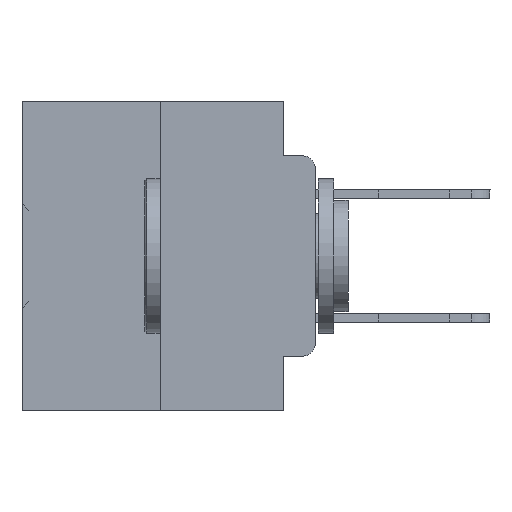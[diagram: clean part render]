
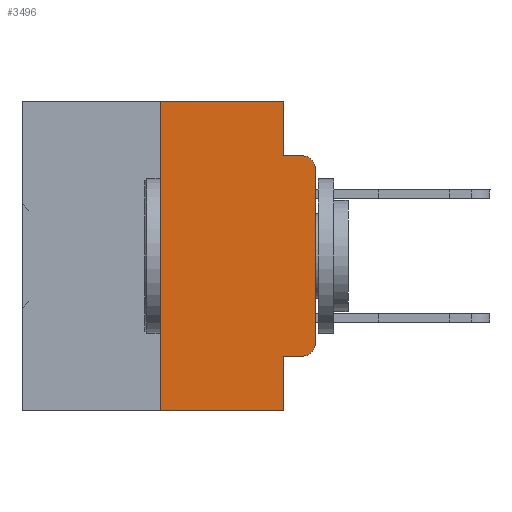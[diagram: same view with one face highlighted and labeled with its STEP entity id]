
A CAD part, left-side view. The second image highlights one B-rep face of the part: STEP entity #3496.
In plain terms, the highlighted planar face has unit normal (-1, 0, 0).
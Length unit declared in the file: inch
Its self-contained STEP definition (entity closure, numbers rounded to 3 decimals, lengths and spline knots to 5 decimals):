
#823 = CARTESIAN_POINT ( 'NONE',  ( 0., 0., -0.1085 ) ) ;
#837 = CARTESIAN_POINT ( 'NONE',  ( 0., 0.02, -0.3915 ) ) ;
#1026 = DIRECTION ( 'NONE',  ( -1., 0., 0. ) ) ;
#1838 = CARTESIAN_POINT ( 'NONE',  ( 0., 0.02, -0.1085 ) ) ;
#2647 = CARTESIAN_POINT ( 'NONE',  ( 0., 0.473, -0.5 ) ) ;
#3114 = ORIENTED_EDGE ( 'NONE', *, *, #18585, .F. ) ;
#3496 = ADVANCED_FACE ( 'NONE', ( #16375 ), #37203, .F. ) ;
#3694 = CARTESIAN_POINT ( 'NONE',  ( 0., 0., 0. ) ) ;
#4032 = CARTESIAN_POINT ( 'NONE',  ( 0., 0., -0.3915 ) ) ;
#4084 = DIRECTION ( 'NONE',  ( 0., 0., 1. ) ) ;
#5084 = CARTESIAN_POINT ( 'NONE',  ( 0., 0.051, -0.4115 ) ) ;
#6543 = VERTEX_POINT ( 'NONE', #823 ) ;
#6663 = LINE ( 'NONE', #18977, #31455 ) ;
#6861 = CARTESIAN_POINT ( 'NONE',  ( 0., 0.473, 0. ) ) ;
#6933 = AXIS2_PLACEMENT_3D ( 'NONE', #1838, #16694, #32371 ) ;
#7284 = ORIENTED_EDGE ( 'NONE', *, *, #8769, .T. ) ;
#7446 = LINE ( 'NONE', #3694, #13860 ) ;
#7814 = DIRECTION ( 'NONE',  ( 0., 0., -1. ) ) ;
#7844 = EDGE_CURVE ( 'NONE', #35624, #34643, #15905, .T. ) ;
#8178 = CIRCLE ( 'NONE', #6933, 0.02 ) ;
#8769 = EDGE_CURVE ( 'NONE', #9172, #6543, #7446, .T. ) ;
#9172 = VERTEX_POINT ( 'NONE', #4032 ) ;
#9744 = CARTESIAN_POINT ( 'NONE',  ( 0., 0.051, -0.0885 ) ) ;
#10042 = DIRECTION ( 'NONE',  ( 1., 0., 0. ) ) ;
#10720 = CARTESIAN_POINT ( 'NONE',  ( 0., 0.051, 0. ) ) ;
#10764 = ORIENTED_EDGE ( 'NONE', *, *, #18396, .T. ) ;
#11374 = DIRECTION ( 'NONE',  ( 0., -1., 0. ) ) ;
#12524 = EDGE_LOOP ( 'NONE', ( #7284, #24530, #14257, #33137, #19031, #15318, #31557, #3114, #10764, #33323 ) ) ;
#12937 = CARTESIAN_POINT ( 'NONE',  ( 0., 0.25, 0. ) ) ;
#13725 = CARTESIAN_POINT ( 'NONE',  ( 0., 0.02, -0.4115 ) ) ;
#13860 = VECTOR ( 'NONE', #15789, 39.37008 ) ;
#14257 = ORIENTED_EDGE ( 'NONE', *, *, #7844, .F. ) ;
#15318 = ORIENTED_EDGE ( 'NONE', *, *, #29337, .F. ) ;
#15789 = DIRECTION ( 'NONE',  ( 0., 0., 1. ) ) ;
#15905 = LINE ( 'NONE', #9744, #36147 ) ;
#16375 = FACE_OUTER_BOUND ( 'NONE', #12524, .T. ) ;
#16694 = DIRECTION ( 'NONE',  ( -1., 0., 0. ) ) ;
#17138 = LINE ( 'NONE', #2647, #18107 ) ;
#17181 = DIRECTION ( 'NONE',  ( 0., -1., 0. ) ) ;
#17596 = AXIS2_PLACEMENT_3D ( 'NONE', #6861, #10042, #22510 ) ;
#17757 = LINE ( 'NONE', #23292, #18221 ) ;
#17761 = LINE ( 'NONE', #5084, #26899 ) ;
#18107 = VECTOR ( 'NONE', #11374, 39.37008 ) ;
#18221 = VECTOR ( 'NONE', #29862, 39.37008 ) ;
#18396 = EDGE_CURVE ( 'NONE', #38470, #26795, #17761, .T. ) ;
#18585 = EDGE_CURVE ( 'NONE', #38470, #37233, #36203, .T. ) ;
#18687 = CARTESIAN_POINT ( 'NONE',  ( 0., 0.25, -0.5 ) ) ;
#18888 = DIRECTION ( 'NONE',  ( 0., 0., -1. ) ) ;
#18977 = CARTESIAN_POINT ( 'NONE',  ( 0., 0.25, 0. ) ) ;
#19031 = ORIENTED_EDGE ( 'NONE', *, *, #28865, .F. ) ;
#21509 = VERTEX_POINT ( 'NONE', #28839 ) ;
#21600 = CIRCLE ( 'NONE', #32363, 0.02 ) ;
#22486 = VECTOR ( 'NONE', #7814, 39.37008 ) ;
#22510 = DIRECTION ( 'NONE',  ( 0., 0., -1. ) ) ;
#22806 = DIRECTION ( 'NONE',  ( 0., 0., -1. ) ) ;
#23292 = CARTESIAN_POINT ( 'NONE',  ( 0., 0.473, 0. ) ) ;
#23345 = VECTOR ( 'NONE', #22806, 39.37008 ) ;
#24530 = ORIENTED_EDGE ( 'NONE', *, *, #35456, .T. ) ;
#25070 = EDGE_CURVE ( 'NONE', #26593, #37233, #17138, .T. ) ;
#26593 = VERTEX_POINT ( 'NONE', #18687 ) ;
#26779 = CARTESIAN_POINT ( 'NONE',  ( 0., 0.051, -0.0885 ) ) ;
#26795 = VERTEX_POINT ( 'NONE', #13725 ) ;
#26899 = VECTOR ( 'NONE', #17181, 39.37008 ) ;
#28142 = CARTESIAN_POINT ( 'NONE',  ( 0., 0.02, -0.0885 ) ) ;
#28568 = LINE ( 'NONE', #10720, #23345 ) ;
#28839 = CARTESIAN_POINT ( 'NONE',  ( 0., 0.051, 0. ) ) ;
#28865 = EDGE_CURVE ( 'NONE', #35377, #21509, #17757, .T. ) ;
#29337 = EDGE_CURVE ( 'NONE', #26593, #35377, #6663, .T. ) ;
#29862 = DIRECTION ( 'NONE',  ( 0., -1., 0. ) ) ;
#31455 = VECTOR ( 'NONE', #4084, 39.37008 ) ;
#31557 = ORIENTED_EDGE ( 'NONE', *, *, #25070, .T. ) ;
#31931 = CARTESIAN_POINT ( 'NONE',  ( 0., 0.051, -0.5 ) ) ;
#32363 = AXIS2_PLACEMENT_3D ( 'NONE', #837, #1026, #18888 ) ;
#32371 = DIRECTION ( 'NONE',  ( 0., 0., -1. ) ) ;
#33137 = ORIENTED_EDGE ( 'NONE', *, *, #37305, .F. ) ;
#33221 = CARTESIAN_POINT ( 'NONE',  ( 0., 0.051, 0. ) ) ;
#33323 = ORIENTED_EDGE ( 'NONE', *, *, #34027, .T. ) ;
#34027 = EDGE_CURVE ( 'NONE', #26795, #9172, #21600, .T. ) ;
#34274 = CARTESIAN_POINT ( 'NONE',  ( 0., 0.051, -0.4115 ) ) ;
#34643 = VERTEX_POINT ( 'NONE', #28142 ) ;
#35377 = VERTEX_POINT ( 'NONE', #12937 ) ;
#35456 = EDGE_CURVE ( 'NONE', #6543, #34643, #8178, .T. ) ;
#35624 = VERTEX_POINT ( 'NONE', #26779 ) ;
#36147 = VECTOR ( 'NONE', #36733, 39.37008 ) ;
#36203 = LINE ( 'NONE', #33221, #22486 ) ;
#36733 = DIRECTION ( 'NONE',  ( 0., -1., 0. ) ) ;
#37203 = PLANE ( 'NONE',  #17596 ) ;
#37233 = VERTEX_POINT ( 'NONE', #31931 ) ;
#37305 = EDGE_CURVE ( 'NONE', #21509, #35624, #28568, .T. ) ;
#38470 = VERTEX_POINT ( 'NONE', #34274 ) ;
